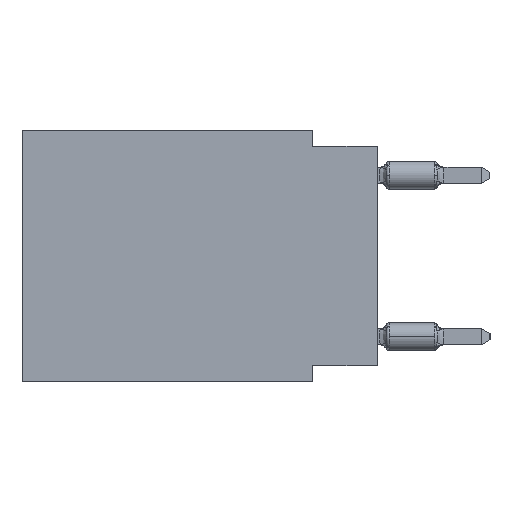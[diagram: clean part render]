
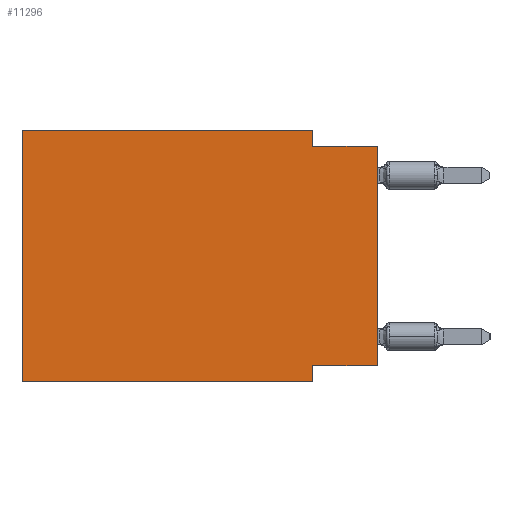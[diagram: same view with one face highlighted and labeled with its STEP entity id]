
A CAD part, left-side view. The second image highlights one B-rep face of the part: STEP entity #11296.
In plain terms, the highlighted planar face has unit normal (-1, 0, 0).
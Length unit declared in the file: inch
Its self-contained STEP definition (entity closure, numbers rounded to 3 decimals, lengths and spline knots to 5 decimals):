
#123 = DIRECTION ( 'NONE',  ( 0., 0., -1. ) ) ;
#290 = FACE_OUTER_BOUND ( 'NONE', #6109, .T. ) ;
#314 = VERTEX_POINT ( 'NONE', #4501 ) ;
#388 = EDGE_CURVE ( 'NONE', #10954, #22852, #17738, .T. ) ;
#708 = VECTOR ( 'NONE', #14105, 39.37008 ) ;
#904 = AXIS2_PLACEMENT_3D ( 'NONE', #10089, #4855, #123 ) ;
#1296 = DIRECTION ( 'NONE',  ( 0., -1., 0. ) ) ;
#1433 = LINE ( 'NONE', #11065, #29389 ) ;
#1523 = LINE ( 'NONE', #6702, #4286 ) ;
#1784 = CARTESIAN_POINT ( 'NONE',  ( 0., 0.55, 0. ) ) ;
#3975 = CARTESIAN_POINT ( 'NONE',  ( 0., 0.55, -0.39 ) ) ;
#4148 = DIRECTION ( 'NONE',  ( 0., 0., 1. ) ) ;
#4286 = VECTOR ( 'NONE', #27871, 39.37008 ) ;
#4501 = CARTESIAN_POINT ( 'NONE',  ( 0., 0., -0.365 ) ) ;
#4855 = DIRECTION ( 'NONE',  ( 1., 0., 0. ) ) ;
#4944 = LINE ( 'NONE', #26399, #708 ) ;
#5128 = ORIENTED_EDGE ( 'NONE', *, *, #5717, .F. ) ;
#5450 = VECTOR ( 'NONE', #15848, 39.37008 ) ;
#5717 = EDGE_CURVE ( 'NONE', #18762, #16942, #18526, .T. ) ;
#6109 = EDGE_LOOP ( 'NONE', ( #28958, #5128, #21488, #21123, #21760, #9952, #10965, #21518 ) ) ;
#6212 = CARTESIAN_POINT ( 'NONE',  ( 0., 0., 0. ) ) ;
#6702 = CARTESIAN_POINT ( 'NONE',  ( 0., 0.1, 0. ) ) ;
#7677 = VERTEX_POINT ( 'NONE', #20213 ) ;
#7767 = VECTOR ( 'NONE', #28129, 39.37008 ) ;
#9155 = VERTEX_POINT ( 'NONE', #28252 ) ;
#9952 = ORIENTED_EDGE ( 'NONE', *, *, #388, .T. ) ;
#10008 = CARTESIAN_POINT ( 'NONE',  ( 0., 0.55, -0.39 ) ) ;
#10089 = CARTESIAN_POINT ( 'NONE',  ( 0., 0.55, 0. ) ) ;
#10954 = VERTEX_POINT ( 'NONE', #10008 ) ;
#10965 = ORIENTED_EDGE ( 'NONE', *, *, #30102, .F. ) ;
#11065 = CARTESIAN_POINT ( 'NONE',  ( 0., 0.1, -0.39 ) ) ;
#11296 = ADVANCED_FACE ( 'NONE', ( #290 ), #19879, .F. ) ;
#11721 = CARTESIAN_POINT ( 'NONE',  ( 0., 0.1, -0.39 ) ) ;
#14105 = DIRECTION ( 'NONE',  ( 0., 1., 0. ) ) ;
#14551 = EDGE_CURVE ( 'NONE', #314, #9155, #4944, .T. ) ;
#14899 = LINE ( 'NONE', #15353, #29691 ) ;
#15353 = CARTESIAN_POINT ( 'NONE',  ( 0., 0.55, 0. ) ) ;
#15848 = DIRECTION ( 'NONE',  ( 0., 0., 1. ) ) ;
#16150 = VERTEX_POINT ( 'NONE', #28903 ) ;
#16376 = VECTOR ( 'NONE', #1296, 39.37008 ) ;
#16942 = VERTEX_POINT ( 'NONE', #29592 ) ;
#17738 = LINE ( 'NONE', #3975, #16376 ) ;
#18526 = LINE ( 'NONE', #25614, #7767 ) ;
#18762 = VERTEX_POINT ( 'NONE', #27769 ) ;
#19879 = PLANE ( 'NONE',  #904 ) ;
#20213 = CARTESIAN_POINT ( 'NONE',  ( 0., 0.55, 0. ) ) ;
#21094 = EDGE_CURVE ( 'NONE', #16150, #18762, #1523, .T. ) ;
#21123 = ORIENTED_EDGE ( 'NONE', *, *, #22957, .F. ) ;
#21488 = ORIENTED_EDGE ( 'NONE', *, *, #21094, .F. ) ;
#21518 = ORIENTED_EDGE ( 'NONE', *, *, #14551, .F. ) ;
#21605 = EDGE_CURVE ( 'NONE', #314, #16942, #28146, .T. ) ;
#21760 = ORIENTED_EDGE ( 'NONE', *, *, #30852, .F. ) ;
#22852 = VERTEX_POINT ( 'NONE', #11721 ) ;
#22957 = EDGE_CURVE ( 'NONE', #7677, #16150, #14899, .T. ) ;
#23892 = VECTOR ( 'NONE', #4148, 39.37008 ) ;
#25314 = LINE ( 'NONE', #1784, #23892 ) ;
#25614 = CARTESIAN_POINT ( 'NONE',  ( 0., 0., -0.025 ) ) ;
#26399 = CARTESIAN_POINT ( 'NONE',  ( 0., 0., -0.365 ) ) ;
#27492 = DIRECTION ( 'NONE',  ( 0., -1., 0. ) ) ;
#27769 = CARTESIAN_POINT ( 'NONE',  ( 0., 0.1, -0.025 ) ) ;
#27871 = DIRECTION ( 'NONE',  ( 0., 0., -1. ) ) ;
#28129 = DIRECTION ( 'NONE',  ( 0., -1., 0. ) ) ;
#28146 = LINE ( 'NONE', #6212, #5450 ) ;
#28252 = CARTESIAN_POINT ( 'NONE',  ( 0., 0.1, -0.365 ) ) ;
#28903 = CARTESIAN_POINT ( 'NONE',  ( 0., 0.1, 0. ) ) ;
#28958 = ORIENTED_EDGE ( 'NONE', *, *, #21605, .T. ) ;
#29389 = VECTOR ( 'NONE', #30291, 39.37008 ) ;
#29592 = CARTESIAN_POINT ( 'NONE',  ( 0., 0., -0.025 ) ) ;
#29691 = VECTOR ( 'NONE', #27492, 39.37008 ) ;
#30102 = EDGE_CURVE ( 'NONE', #9155, #22852, #1433, .T. ) ;
#30291 = DIRECTION ( 'NONE',  ( 0., 0., -1. ) ) ;
#30852 = EDGE_CURVE ( 'NONE', #10954, #7677, #25314, .T. ) ;
